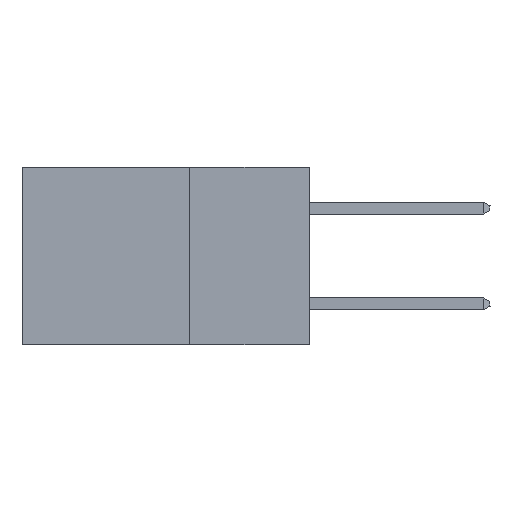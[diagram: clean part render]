
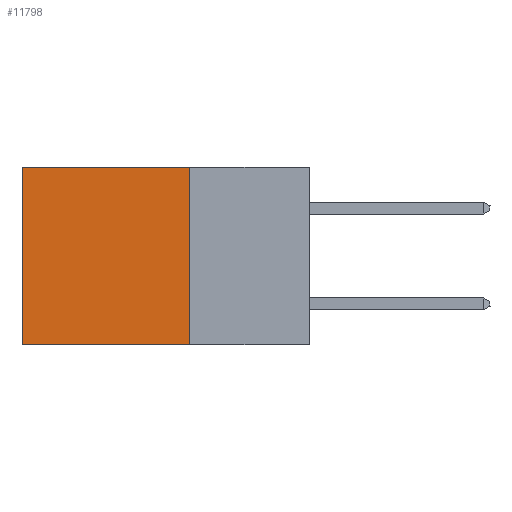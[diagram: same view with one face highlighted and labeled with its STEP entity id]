
A CAD part, left-side view. The second image highlights one B-rep face of the part: STEP entity #11798.
In plain terms, the highlighted planar face has unit normal (-1, 0, 0).
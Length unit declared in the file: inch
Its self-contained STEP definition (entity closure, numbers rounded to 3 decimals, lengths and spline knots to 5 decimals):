
#94 = CARTESIAN_POINT ( 'NONE',  ( 0.2875, 0.25, 0. ) ) ;
#572 = ORIENTED_EDGE ( 'NONE', *, *, #6457, .T. ) ;
#870 = VECTOR ( 'NONE', #3149, 39.37008 ) ;
#2151 = VECTOR ( 'NONE', #12340, 39.37008 ) ;
#2324 = DIRECTION ( 'NONE',  ( 1., 0., 0. ) ) ;
#2613 = VECTOR ( 'NONE', #2779, 39.37008 ) ;
#2779 = DIRECTION ( 'NONE',  ( 0., 1., 0. ) ) ;
#2879 = LINE ( 'NONE', #94, #7217 ) ;
#3149 = DIRECTION ( 'NONE',  ( 0., 0., -1. ) ) ;
#3317 = CARTESIAN_POINT ( 'NONE',  ( 0.2875, 0.25, -0.37 ) ) ;
#3382 = DIRECTION ( 'NONE',  ( 0., 0., -1. ) ) ;
#3598 = ORIENTED_EDGE ( 'NONE', *, *, #13401, .F. ) ;
#4191 = FACE_OUTER_BOUND ( 'NONE', #11343, .T. ) ;
#4323 = CARTESIAN_POINT ( 'NONE',  ( 0.2875, 0.25, -0.37 ) ) ;
#6440 = CARTESIAN_POINT ( 'NONE',  ( 0.2875, 0.25, 0. ) ) ;
#6457 = EDGE_CURVE ( 'NONE', #8586, #10087, #8795, .T. ) ;
#6471 = LINE ( 'NONE', #4323, #2613 ) ;
#6603 = CARTESIAN_POINT ( 'NONE',  ( 0.2875, 0.25, 0. ) ) ;
#6858 = VERTEX_POINT ( 'NONE', #6603 ) ;
#6899 = LINE ( 'NONE', #9287, #870 ) ;
#7115 = ORIENTED_EDGE ( 'NONE', *, *, #13399, .T. ) ;
#7217 = VECTOR ( 'NONE', #10486, 39.37008 ) ;
#7764 = VERTEX_POINT ( 'NONE', #3317 ) ;
#8311 = CARTESIAN_POINT ( 'NONE',  ( 0.2875, 0.6, 0. ) ) ;
#8586 = VERTEX_POINT ( 'NONE', #10439 ) ;
#8620 = CARTESIAN_POINT ( 'NONE',  ( 0.2875, 0.6, -0.37 ) ) ;
#8795 = LINE ( 'NONE', #8311, #2151 ) ;
#8917 = ORIENTED_EDGE ( 'NONE', *, *, #11321, .F. ) ;
#9287 = CARTESIAN_POINT ( 'NONE',  ( 0.2875, 0.25, 0. ) ) ;
#10087 = VERTEX_POINT ( 'NONE', #8620 ) ;
#10439 = CARTESIAN_POINT ( 'NONE',  ( 0.2875, 0.6, 0. ) ) ;
#10486 = DIRECTION ( 'NONE',  ( 0., 1., 0. ) ) ;
#11321 = EDGE_CURVE ( 'NONE', #7764, #10087, #6471, .T. ) ;
#11343 = EDGE_LOOP ( 'NONE', ( #572, #8917, #3598, #7115 ) ) ;
#11798 = ADVANCED_FACE ( 'NONE', ( #4191 ), #12655, .F. ) ;
#12340 = DIRECTION ( 'NONE',  ( 0., 0., -1. ) ) ;
#12655 = PLANE ( 'NONE',  #12746 ) ;
#12746 = AXIS2_PLACEMENT_3D ( 'NONE', #6440, #2324, #3382 ) ;
#13399 = EDGE_CURVE ( 'NONE', #6858, #8586, #2879, .T. ) ;
#13401 = EDGE_CURVE ( 'NONE', #6858, #7764, #6899, .T. ) ;
